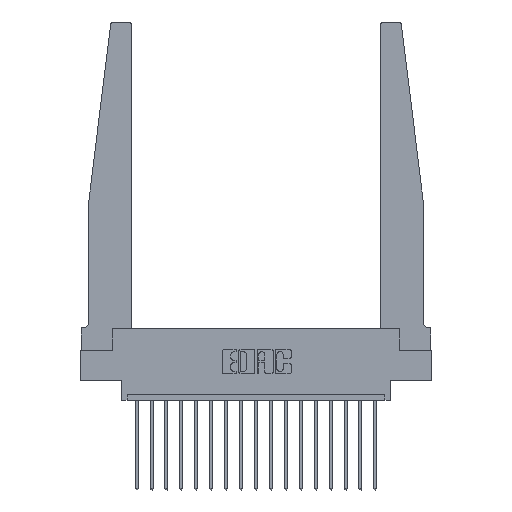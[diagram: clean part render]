
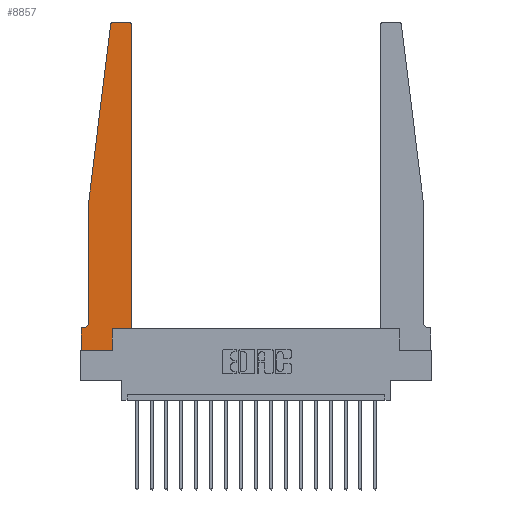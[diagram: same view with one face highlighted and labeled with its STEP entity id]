
A CAD part, top view. The second image highlights one B-rep face of the part: STEP entity #8857.
In plain terms, the highlighted planar face has unit normal (0, 0, 1).
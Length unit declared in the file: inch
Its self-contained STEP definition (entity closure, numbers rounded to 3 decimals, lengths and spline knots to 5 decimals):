
#123 = VECTOR ( 'NONE', #4578, 39.37008 ) ;
#385 = VERTEX_POINT ( 'NONE', #822 ) ;
#822 = CARTESIAN_POINT ( 'NONE',  ( 0.2605, 0.18, 0.37 ) ) ;
#1068 = DIRECTION ( 'NONE',  ( -1., 0., 0. ) ) ;
#1452 = VERTEX_POINT ( 'NONE', #16276 ) ;
#1495 = CARTESIAN_POINT ( 'NONE',  ( 0.065, 0.2375, 0.37 ) ) ;
#1666 = LINE ( 'NONE', #3392, #7358 ) ;
#1736 = EDGE_CURVE ( 'NONE', #385, #1452, #16527, .T. ) ;
#1739 = DIRECTION ( 'NONE',  ( 1., 0., 0. ) ) ;
#1749 = CARTESIAN_POINT ( 'NONE',  ( 0.2605, 0., 0.37 ) ) ;
#1763 = EDGE_CURVE ( 'NONE', #6936, #4990, #5108, .T. ) ;
#2244 = LINE ( 'NONE', #2895, #11907 ) ;
#2536 = CARTESIAN_POINT ( 'NONE',  ( 0.395, 2.75, 0.37 ) ) ;
#2717 = EDGE_CURVE ( 'NONE', #8306, #12858, #13779, .T. ) ;
#2751 = ORIENTED_EDGE ( 'NONE', *, *, #11289, .T. ) ;
#2895 = CARTESIAN_POINT ( 'NONE',  ( 0.425, 0.18, 0.37 ) ) ;
#2915 = CARTESIAN_POINT ( 'NONE',  ( 0., 0.1875, 0.37 ) ) ;
#3194 = DIRECTION ( 'NONE',  ( -1., 0., 0. ) ) ;
#3392 = CARTESIAN_POINT ( 'NONE',  ( 0.065, 0.1875, 0.37 ) ) ;
#3928 = LINE ( 'NONE', #7559, #12415 ) ;
#3984 = EDGE_CURVE ( 'NONE', #4990, #7449, #7324, .T. ) ;
#4060 = CARTESIAN_POINT ( 'NONE',  ( 0.2605, 0.18, 0.37 ) ) ;
#4578 = DIRECTION ( 'NONE',  ( 0., -1., 0. ) ) ;
#4701 = CARTESIAN_POINT ( 'NONE',  ( 0.27653, 2.75, 0.37 ) ) ;
#4761 = DIRECTION ( 'NONE',  ( 1., 0., 0. ) ) ;
#4990 = VERTEX_POINT ( 'NONE', #6253 ) ;
#5108 = LINE ( 'NONE', #16480, #15601 ) ;
#5633 = DIRECTION ( 'NONE',  ( 0., 1., 0. ) ) ;
#5851 = CARTESIAN_POINT ( 'NONE',  ( 0., 0.1875, 0.37 ) ) ;
#6188 = VECTOR ( 'NONE', #14074, 39.37008 ) ;
#6253 = CARTESIAN_POINT ( 'NONE',  ( 0., 0., 0.37 ) ) ;
#6858 = EDGE_CURVE ( 'NONE', #13423, #12758, #10936, .T. ) ;
#6892 = DIRECTION ( 'NONE',  ( 0., 0., 1. ) ) ;
#6936 = VERTEX_POINT ( 'NONE', #2915 ) ;
#6995 = CARTESIAN_POINT ( 'NONE',  ( 0.395, 2.72, 0.37 ) ) ;
#7273 = CARTESIAN_POINT ( 'NONE',  ( 0.24675, 2.72367, 0.37 ) ) ;
#7324 = LINE ( 'NONE', #14015, #6188 ) ;
#7358 = VECTOR ( 'NONE', #10725, 39.37008 ) ;
#7449 = VERTEX_POINT ( 'NONE', #1749 ) ;
#7473 = ORIENTED_EDGE ( 'NONE', *, *, #6858, .T. ) ;
#7559 = CARTESIAN_POINT ( 'NONE',  ( 0.065, 1.25, 0.37 ) ) ;
#7643 = AXIS2_PLACEMENT_3D ( 'NONE', #6995, #17168, #9767 ) ;
#7854 = AXIS2_PLACEMENT_3D ( 'NONE', #11228, #6892, #8765 ) ;
#7855 = VECTOR ( 'NONE', #3194, 39.37008 ) ;
#8306 = VERTEX_POINT ( 'NONE', #4701 ) ;
#8512 = VERTEX_POINT ( 'NONE', #13417 ) ;
#8621 = ORIENTED_EDGE ( 'NONE', *, *, #14215, .T. ) ;
#8765 = DIRECTION ( 'NONE',  ( 1., 0., 0. ) ) ;
#8857 = ADVANCED_FACE ( 'NONE', ( #10883 ), #8866, .T. ) ;
#8866 = PLANE ( 'NONE',  #16226 ) ;
#9153 = DIRECTION ( 'NONE',  ( -0.122, -0.992, 0. ) ) ;
#9202 = EDGE_CURVE ( 'NONE', #14374, #13423, #9471, .T. ) ;
#9434 = EDGE_CURVE ( 'NONE', #11351, #8306, #9708, .T. ) ;
#9471 = LINE ( 'NONE', #10294, #123 ) ;
#9621 = DIRECTION ( 'NONE',  ( 0., 0., -1. ) ) ;
#9708 = LINE ( 'NONE', #13289, #7855 ) ;
#9767 = DIRECTION ( 'NONE',  ( 1., 0., 0. ) ) ;
#9795 = EDGE_CURVE ( 'NONE', #7449, #385, #14920, .T. ) ;
#10294 = CARTESIAN_POINT ( 'NONE',  ( 0.065, 1.25, 0.37 ) ) ;
#10511 = CIRCLE ( 'NONE', #7643, 0.03 ) ;
#10522 = DIRECTION ( 'NONE',  ( 0., 0., 1. ) ) ;
#10725 = DIRECTION ( 'NONE',  ( -1., 0., 0. ) ) ;
#10734 = EDGE_LOOP ( 'NONE', ( #12312, #13476, #8621, #14753, #7473, #2751, #17850, #12582, #18601, #11234, #17283, #15228 ) ) ;
#10763 = CARTESIAN_POINT ( 'NONE',  ( 0.015, 0.1875, 0.37 ) ) ;
#10774 = DIRECTION ( 'NONE',  ( 0., -1., 0. ) ) ;
#10883 = FACE_OUTER_BOUND ( 'NONE', #10734, .T. ) ;
#10936 = CIRCLE ( 'NONE', #13306, 0.05 ) ;
#11228 = CARTESIAN_POINT ( 'NONE',  ( 0.27653, 2.72, 0.37 ) ) ;
#11234 = ORIENTED_EDGE ( 'NONE', *, *, #1736, .T. ) ;
#11289 = EDGE_CURVE ( 'NONE', #12758, #6936, #1666, .T. ) ;
#11351 = VERTEX_POINT ( 'NONE', #2536 ) ;
#11907 = VECTOR ( 'NONE', #18832, 39.37008 ) ;
#12304 = CARTESIAN_POINT ( 'NONE',  ( 0.425, 0.18, 0.37 ) ) ;
#12312 = ORIENTED_EDGE ( 'NONE', *, *, #9434, .T. ) ;
#12415 = VECTOR ( 'NONE', #9153, 39.37008 ) ;
#12582 = ORIENTED_EDGE ( 'NONE', *, *, #3984, .T. ) ;
#12758 = VERTEX_POINT ( 'NONE', #10763 ) ;
#12858 = VERTEX_POINT ( 'NONE', #7273 ) ;
#13289 = CARTESIAN_POINT ( 'NONE',  ( 0.25, 2.75, 0.37 ) ) ;
#13306 = AXIS2_PLACEMENT_3D ( 'NONE', #18353, #9621, #1068 ) ;
#13417 = CARTESIAN_POINT ( 'NONE',  ( 0.425, 2.72, 0.37 ) ) ;
#13423 = VERTEX_POINT ( 'NONE', #1495 ) ;
#13476 = ORIENTED_EDGE ( 'NONE', *, *, #2717, .T. ) ;
#13572 = VECTOR ( 'NONE', #5633, 39.37008 ) ;
#13779 = CIRCLE ( 'NONE', #7854, 0.03 ) ;
#14015 = CARTESIAN_POINT ( 'NONE',  ( 0., 0., 0.37 ) ) ;
#14074 = DIRECTION ( 'NONE',  ( 1., 0., 0. ) ) ;
#14215 = EDGE_CURVE ( 'NONE', #12858, #14374, #3928, .T. ) ;
#14374 = VERTEX_POINT ( 'NONE', #14589 ) ;
#14589 = CARTESIAN_POINT ( 'NONE',  ( 0.065, 1.25, 0.37 ) ) ;
#14753 = ORIENTED_EDGE ( 'NONE', *, *, #9202, .T. ) ;
#14920 = LINE ( 'NONE', #4060, #13572 ) ;
#15228 = ORIENTED_EDGE ( 'NONE', *, *, #16031, .T. ) ;
#15601 = VECTOR ( 'NONE', #10774, 39.37008 ) ;
#16031 = EDGE_CURVE ( 'NONE', #8512, #11351, #10511, .T. ) ;
#16226 = AXIS2_PLACEMENT_3D ( 'NONE', #5851, #10522, #1739 ) ;
#16276 = CARTESIAN_POINT ( 'NONE',  ( 0.425, 0.18, 0.37 ) ) ;
#16480 = CARTESIAN_POINT ( 'NONE',  ( 0., 0., 0.37 ) ) ;
#16527 = LINE ( 'NONE', #12304, #17391 ) ;
#16552 = EDGE_CURVE ( 'NONE', #1452, #8512, #2244, .T. ) ;
#17168 = DIRECTION ( 'NONE',  ( 0., 0., 1. ) ) ;
#17283 = ORIENTED_EDGE ( 'NONE', *, *, #16552, .T. ) ;
#17391 = VECTOR ( 'NONE', #4761, 39.37008 ) ;
#17850 = ORIENTED_EDGE ( 'NONE', *, *, #1763, .T. ) ;
#18353 = CARTESIAN_POINT ( 'NONE',  ( 0.015, 0.2375, 0.37 ) ) ;
#18601 = ORIENTED_EDGE ( 'NONE', *, *, #9795, .T. ) ;
#18832 = DIRECTION ( 'NONE',  ( 0., 1., 0. ) ) ;
